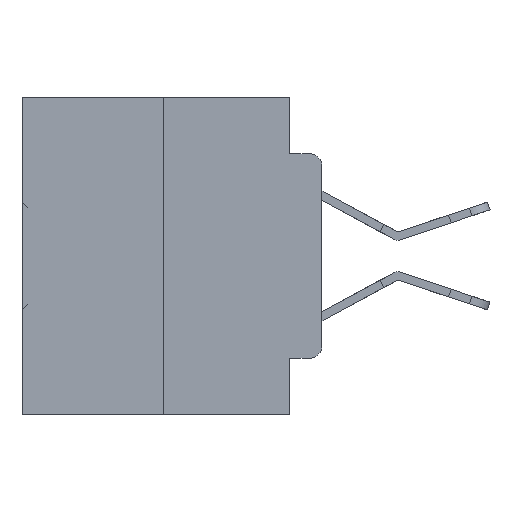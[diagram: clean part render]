
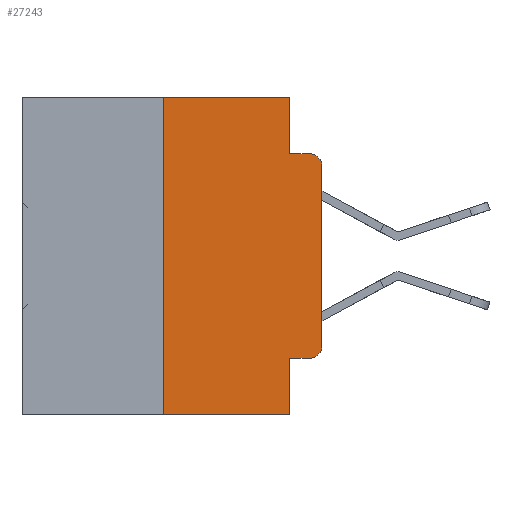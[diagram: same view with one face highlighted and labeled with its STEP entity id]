
A CAD part, left-side view. The second image highlights one B-rep face of the part: STEP entity #27243.
In plain terms, the highlighted planar face has unit normal (-1, 0, 0).
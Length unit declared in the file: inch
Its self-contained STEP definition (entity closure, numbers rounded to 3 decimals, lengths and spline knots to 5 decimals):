
#1613 = CARTESIAN_POINT ( 'NONE',  ( 0., 0., -0.3915 ) ) ;
#1938 = LINE ( 'NONE', #3354, #15481 ) ;
#2562 = CARTESIAN_POINT ( 'NONE',  ( 0., 0., 0. ) ) ;
#3354 = CARTESIAN_POINT ( 'NONE',  ( 0., 0.473, -0.5 ) ) ;
#3358 = DIRECTION ( 'NONE',  ( -1., 0., 0. ) ) ;
#4174 = VERTEX_POINT ( 'NONE', #1613 ) ;
#4300 = DIRECTION ( 'NONE',  ( 0., 0., -1. ) ) ;
#4429 = CARTESIAN_POINT ( 'NONE',  ( 0., 0.051, 0. ) ) ;
#4494 = VERTEX_POINT ( 'NONE', #14663 ) ;
#4903 = VERTEX_POINT ( 'NONE', #13655 ) ;
#5311 = EDGE_LOOP ( 'NONE', ( #21224, #22303, #29253, #35728, #26130, #28830, #35756, #29444, #8394, #33726 ) ) ;
#5380 = VERTEX_POINT ( 'NONE', #20693 ) ;
#5539 = DIRECTION ( 'NONE',  ( 0., 0., -1. ) ) ;
#5703 = CARTESIAN_POINT ( 'NONE',  ( 0., 0.051, -0.4115 ) ) ;
#6059 = LINE ( 'NONE', #4429, #29442 ) ;
#6284 = CARTESIAN_POINT ( 'NONE',  ( 0., 0.02, -0.4115 ) ) ;
#6860 = VECTOR ( 'NONE', #8119, 39.37008 ) ;
#7287 = CARTESIAN_POINT ( 'NONE',  ( 0., 0.051, -0.0885 ) ) ;
#8006 = DIRECTION ( 'NONE',  ( 0., -1., 0. ) ) ;
#8119 = DIRECTION ( 'NONE',  ( 0., 0., 1. ) ) ;
#8238 = DIRECTION ( 'NONE',  ( 0., 0., 1. ) ) ;
#8394 = ORIENTED_EDGE ( 'NONE', *, *, #35265, .T. ) ;
#8676 = DIRECTION ( 'NONE',  ( 0., -1., 0. ) ) ;
#8867 = LINE ( 'NONE', #19716, #17366 ) ;
#9584 = CARTESIAN_POINT ( 'NONE',  ( 0., 0.051, 0. ) ) ;
#10284 = CARTESIAN_POINT ( 'NONE',  ( 0., 0.473, 0. ) ) ;
#10694 = VERTEX_POINT ( 'NONE', #6284 ) ;
#10808 = DIRECTION ( 'NONE',  ( 0., -1., 0. ) ) ;
#10814 = VERTEX_POINT ( 'NONE', #7287 ) ;
#11216 = AXIS2_PLACEMENT_3D ( 'NONE', #32718, #30210, #33213 ) ;
#13029 = CARTESIAN_POINT ( 'NONE',  ( 0., 0.473, 0. ) ) ;
#13041 = LINE ( 'NONE', #33614, #32283 ) ;
#13318 = AXIS2_PLACEMENT_3D ( 'NONE', #17815, #3358, #17446 ) ;
#13546 = CARTESIAN_POINT ( 'NONE',  ( 0., 0.25, 0. ) ) ;
#13655 = CARTESIAN_POINT ( 'NONE',  ( 0., 0.25, 0. ) ) ;
#14156 = EDGE_CURVE ( 'NONE', #4903, #25425, #21888, .T. ) ;
#14408 = VERTEX_POINT ( 'NONE', #5703 ) ;
#14663 = CARTESIAN_POINT ( 'NONE',  ( 0., 0.051, -0.5 ) ) ;
#14851 = EDGE_CURVE ( 'NONE', #14408, #4494, #8867, .T. ) ;
#15481 = VECTOR ( 'NONE', #8676, 39.37008 ) ;
#15705 = CARTESIAN_POINT ( 'NONE',  ( 0., 0.02, -0.0885 ) ) ;
#16025 = PLANE ( 'NONE',  #20684 ) ;
#16724 = CARTESIAN_POINT ( 'NONE',  ( 0., 0.051, -0.4115 ) ) ;
#17366 = VECTOR ( 'NONE', #5539, 39.37008 ) ;
#17446 = DIRECTION ( 'NONE',  ( 0., 0., -1. ) ) ;
#17815 = CARTESIAN_POINT ( 'NONE',  ( 0., 0.02, -0.3915 ) ) ;
#18061 = LINE ( 'NONE', #2562, #6860 ) ;
#19491 = VECTOR ( 'NONE', #28004, 39.37008 ) ;
#19716 = CARTESIAN_POINT ( 'NONE',  ( 0., 0.051, 0. ) ) ;
#19881 = CIRCLE ( 'NONE', #11216, 0.02 ) ;
#20066 = CARTESIAN_POINT ( 'NONE',  ( 0., 0.25, -0.5 ) ) ;
#20618 = EDGE_CURVE ( 'NONE', #25425, #10814, #6059, .T. ) ;
#20684 = AXIS2_PLACEMENT_3D ( 'NONE', #13029, #27041, #4300 ) ;
#20693 = CARTESIAN_POINT ( 'NONE',  ( 0., 0., -0.1085 ) ) ;
#20730 = EDGE_CURVE ( 'NONE', #28125, #4903, #32085, .T. ) ;
#21224 = ORIENTED_EDGE ( 'NONE', *, *, #36374, .T. ) ;
#21474 = EDGE_CURVE ( 'NONE', #28125, #4494, #1938, .T. ) ;
#21819 = EDGE_CURVE ( 'NONE', #5380, #34651, #19881, .T. ) ;
#21876 = DIRECTION ( 'NONE',  ( 0., 0., -1. ) ) ;
#21888 = LINE ( 'NONE', #10284, #23713 ) ;
#22156 = CIRCLE ( 'NONE', #13318, 0.02 ) ;
#22303 = ORIENTED_EDGE ( 'NONE', *, *, #21819, .T. ) ;
#22671 = VECTOR ( 'NONE', #8238, 39.37008 ) ;
#23713 = VECTOR ( 'NONE', #8006, 39.37008 ) ;
#23949 = EDGE_CURVE ( 'NONE', #10814, #34651, #13041, .T. ) ;
#25425 = VERTEX_POINT ( 'NONE', #9584 ) ;
#26130 = ORIENTED_EDGE ( 'NONE', *, *, #14156, .F. ) ;
#27041 = DIRECTION ( 'NONE',  ( 1., 0., 0. ) ) ;
#27243 = ADVANCED_FACE ( 'NONE', ( #31317 ), #16025, .F. ) ;
#28004 = DIRECTION ( 'NONE',  ( 0., -1., 0. ) ) ;
#28125 = VERTEX_POINT ( 'NONE', #20066 ) ;
#28830 = ORIENTED_EDGE ( 'NONE', *, *, #20730, .F. ) ;
#29253 = ORIENTED_EDGE ( 'NONE', *, *, #23949, .F. ) ;
#29442 = VECTOR ( 'NONE', #21876, 39.37008 ) ;
#29444 = ORIENTED_EDGE ( 'NONE', *, *, #14851, .F. ) ;
#30210 = DIRECTION ( 'NONE',  ( -1., 0., 0. ) ) ;
#31317 = FACE_OUTER_BOUND ( 'NONE', #5311, .T. ) ;
#32085 = LINE ( 'NONE', #13546, #22671 ) ;
#32283 = VECTOR ( 'NONE', #10808, 39.37008 ) ;
#32528 = LINE ( 'NONE', #16724, #19491 ) ;
#32718 = CARTESIAN_POINT ( 'NONE',  ( 0., 0.02, -0.1085 ) ) ;
#33213 = DIRECTION ( 'NONE',  ( 0., 0., -1. ) ) ;
#33614 = CARTESIAN_POINT ( 'NONE',  ( 0., 0.051, -0.0885 ) ) ;
#33726 = ORIENTED_EDGE ( 'NONE', *, *, #35442, .T. ) ;
#34651 = VERTEX_POINT ( 'NONE', #15705 ) ;
#35265 = EDGE_CURVE ( 'NONE', #14408, #10694, #32528, .T. ) ;
#35442 = EDGE_CURVE ( 'NONE', #10694, #4174, #22156, .T. ) ;
#35728 = ORIENTED_EDGE ( 'NONE', *, *, #20618, .F. ) ;
#35756 = ORIENTED_EDGE ( 'NONE', *, *, #21474, .T. ) ;
#36374 = EDGE_CURVE ( 'NONE', #4174, #5380, #18061, .T. ) ;
